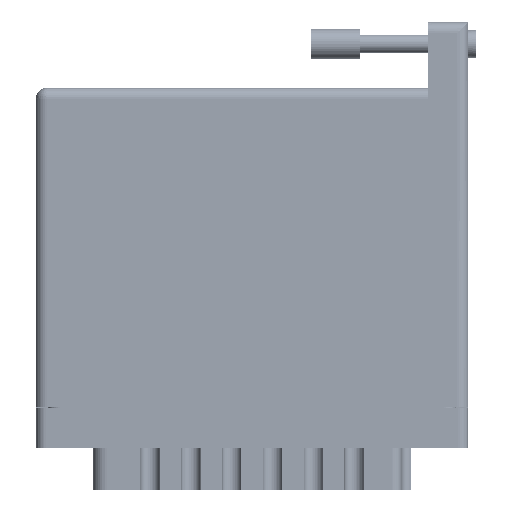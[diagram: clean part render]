
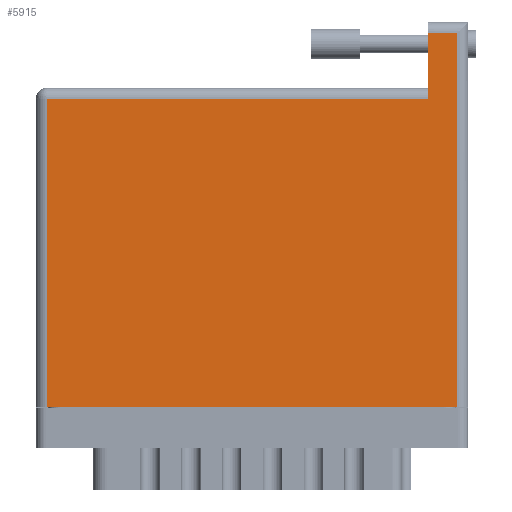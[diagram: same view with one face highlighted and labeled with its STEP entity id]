
A CAD part, front view. The second image highlights one B-rep face of the part: STEP entity #5915.
In plain terms, the highlighted face is planar.
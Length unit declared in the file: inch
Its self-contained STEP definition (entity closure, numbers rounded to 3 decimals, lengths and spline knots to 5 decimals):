
#516 = EDGE_CURVE ( 'NONE', #85616, #58876, #70636, .T. ) ;
#3253 = VECTOR ( 'NONE', #57837, 39.37008 ) ;
#3925 = ORIENTED_EDGE ( 'NONE', *, *, #95529, .T. ) ;
#5311 = CARTESIAN_POINT ( 'NONE',  ( 2.685, 0., 0. ) ) ;
#5915 = ADVANCED_FACE ( 'NONE', ( #84164 ), #10036, .F. ) ;
#8353 = CARTESIAN_POINT ( 'NONE',  ( 2.499, 2.45, 0. ) ) ;
#9449 = VERTEX_POINT ( 'NONE', #5311 ) ;
#9949 = VERTEX_POINT ( 'NONE', #71524 ) ;
#10036 = PLANE ( 'NONE',  #79792 ) ;
#11609 = LINE ( 'NONE', #48204, #84218 ) ;
#12673 = VECTOR ( 'NONE', #83273, 39.37008 ) ;
#13813 = VECTOR ( 'NONE', #28851, 39.37008 ) ;
#15193 = DIRECTION ( 'NONE',  ( -1., 0., 0. ) ) ;
#16096 = EDGE_CURVE ( 'NONE', #9949, #85655, #27883, .T. ) ;
#20279 = CARTESIAN_POINT ( 'NONE',  ( 2.685, 2.45, 0. ) ) ;
#23423 = ORIENTED_EDGE ( 'NONE', *, *, #30407, .T. ) ;
#23525 = EDGE_CURVE ( 'NONE', #52184, #85616, #82785, .T. ) ;
#25795 = VECTOR ( 'NONE', #15193, 39.37008 ) ;
#27883 = LINE ( 'NONE', #83455, #25795 ) ;
#28851 = DIRECTION ( 'NONE',  ( 0., -1., 0. ) ) ;
#29844 = ORIENTED_EDGE ( 'NONE', *, *, #23525, .T. ) ;
#30407 = EDGE_CURVE ( 'NONE', #58876, #9449, #11609, .T. ) ;
#35486 = CARTESIAN_POINT ( 'NONE',  ( 0.07, 0., 0. ) ) ;
#43182 = EDGE_LOOP ( 'NONE', ( #84715, #29844, #54084, #23423, #3925, #43603 ) ) ;
#43603 = ORIENTED_EDGE ( 'NONE', *, *, #16096, .T. ) ;
#44948 = CARTESIAN_POINT ( 'NONE',  ( 0.07, 1.96, 0. ) ) ;
#48061 = DIRECTION ( 'NONE',  ( 0., 0., -1. ) ) ;
#48204 = CARTESIAN_POINT ( 'NONE',  ( 0., 0., 0. ) ) ;
#48210 = CARTESIAN_POINT ( 'NONE',  ( 0.07, 0., 0. ) ) ;
#49167 = CARTESIAN_POINT ( 'NONE',  ( 2.499, 1.96, 0. ) ) ;
#52184 = VERTEX_POINT ( 'NONE', #49167 ) ;
#53518 = CARTESIAN_POINT ( 'NONE',  ( 0., 1.96, 0. ) ) ;
#54084 = ORIENTED_EDGE ( 'NONE', *, *, #516, .T. ) ;
#57837 = DIRECTION ( 'NONE',  ( 0., 1., 0. ) ) ;
#58876 = VERTEX_POINT ( 'NONE', #35486 ) ;
#64659 = EDGE_CURVE ( 'NONE', #85655, #52184, #75161, .T. ) ;
#68558 = CARTESIAN_POINT ( 'NONE',  ( 0., 2.03, 0. ) ) ;
#70636 = LINE ( 'NONE', #48210, #83884 ) ;
#71524 = CARTESIAN_POINT ( 'NONE',  ( 2.685, 2.38, 0. ) ) ;
#75161 = LINE ( 'NONE', #8353, #13813 ) ;
#77331 = DIRECTION ( 'NONE',  ( -1., 0., 0. ) ) ;
#77954 = DIRECTION ( 'NONE',  ( 0., -1., 0. ) ) ;
#79792 = AXIS2_PLACEMENT_3D ( 'NONE', #68558, #48061, #77331 ) ;
#81536 = CARTESIAN_POINT ( 'NONE',  ( 2.499, 2.38, 0. ) ) ;
#82785 = LINE ( 'NONE', #53518, #12673 ) ;
#83273 = DIRECTION ( 'NONE',  ( -1., 0., 0. ) ) ;
#83455 = CARTESIAN_POINT ( 'NONE',  ( 0., 2.38, 0. ) ) ;
#83884 = VECTOR ( 'NONE', #77954, 39.37008 ) ;
#84164 = FACE_OUTER_BOUND ( 'NONE', #43182, .T. ) ;
#84218 = VECTOR ( 'NONE', #85734, 39.37008 ) ;
#84715 = ORIENTED_EDGE ( 'NONE', *, *, #64659, .T. ) ;
#85616 = VERTEX_POINT ( 'NONE', #44948 ) ;
#85655 = VERTEX_POINT ( 'NONE', #81536 ) ;
#85734 = DIRECTION ( 'NONE',  ( 1., 0., 0. ) ) ;
#87104 = LINE ( 'NONE', #20279, #3253 ) ;
#95529 = EDGE_CURVE ( 'NONE', #9449, #9949, #87104, .T. ) ;
